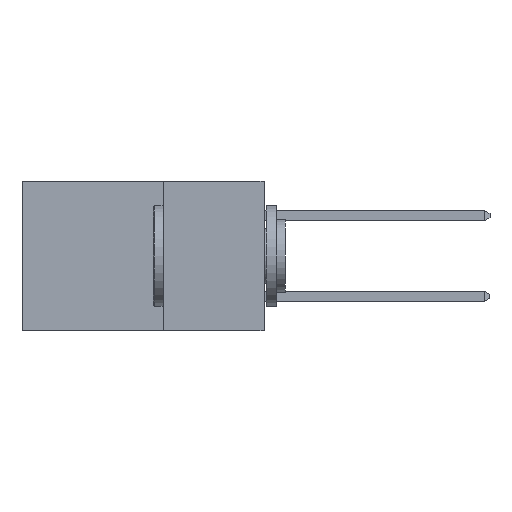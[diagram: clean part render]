
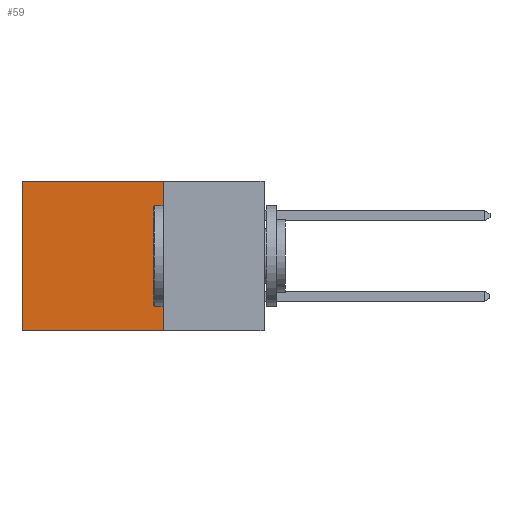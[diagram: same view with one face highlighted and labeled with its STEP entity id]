
A CAD part, left-side view. The second image highlights one B-rep face of the part: STEP entity #59.
In plain terms, the highlighted planar face has unit normal (-1, 0, 0).
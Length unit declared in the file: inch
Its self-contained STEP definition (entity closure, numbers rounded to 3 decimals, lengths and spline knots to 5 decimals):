
#59 = ADVANCED_FACE ( 'NONE', ( #3727 ), #8161, .F. ) ;
#209 = VERTEX_POINT ( 'NONE', #6655 ) ;
#684 = DIRECTION ( 'NONE',  ( 0., 1., 0. ) ) ;
#915 = EDGE_LOOP ( 'NONE', ( #1924, #1939, #1951, #2001 ) ) ;
#956 = VECTOR ( 'NONE', #684, 39.37008 ) ;
#1841 = CARTESIAN_POINT ( 'NONE',  ( 0.298, 0.25, 0. ) ) ;
#1924 = ORIENTED_EDGE ( 'NONE', *, *, #4105, .T. ) ;
#1939 = ORIENTED_EDGE ( 'NONE', *, *, #3051, .F. ) ;
#1951 = ORIENTED_EDGE ( 'NONE', *, *, #7967, .F. ) ;
#2001 = ORIENTED_EDGE ( 'NONE', *, *, #9810, .T. ) ;
#2550 = VECTOR ( 'NONE', #6316, 39.37008 ) ;
#2559 = CARTESIAN_POINT ( 'NONE',  ( 0.298, 0.25, -0.37 ) ) ;
#2726 = VERTEX_POINT ( 'NONE', #8620 ) ;
#3051 = EDGE_CURVE ( 'NONE', #2726, #209, #3172, .T. ) ;
#3147 = LINE ( 'NONE', #5166, #5351 ) ;
#3172 = LINE ( 'NONE', #2559, #956 ) ;
#3714 = AXIS2_PLACEMENT_3D ( 'NONE', #1841, #8182, #6982 ) ;
#3727 = FACE_OUTER_BOUND ( 'NONE', #915, .T. ) ;
#4105 = EDGE_CURVE ( 'NONE', #5704, #209, #6999, .T. ) ;
#4434 = DIRECTION ( 'NONE',  ( 0., 1., 0. ) ) ;
#4798 = LINE ( 'NONE', #9289, #2550 ) ;
#4989 = VECTOR ( 'NONE', #8642, 39.37008 ) ;
#5166 = CARTESIAN_POINT ( 'NONE',  ( 0.298, 0.25, 0. ) ) ;
#5224 = VERTEX_POINT ( 'NONE', #6948 ) ;
#5351 = VECTOR ( 'NONE', #4434, 39.37008 ) ;
#5704 = VERTEX_POINT ( 'NONE', #9781 ) ;
#6316 = DIRECTION ( 'NONE',  ( 0., 0., -1. ) ) ;
#6655 = CARTESIAN_POINT ( 'NONE',  ( 0.298, 0.6, -0.37 ) ) ;
#6948 = CARTESIAN_POINT ( 'NONE',  ( 0.298, 0.25, 0. ) ) ;
#6982 = DIRECTION ( 'NONE',  ( 0., 0., -1. ) ) ;
#6999 = LINE ( 'NONE', #7844, #4989 ) ;
#7844 = CARTESIAN_POINT ( 'NONE',  ( 0.298, 0.6, 0. ) ) ;
#7967 = EDGE_CURVE ( 'NONE', #5224, #2726, #4798, .T. ) ;
#8161 = PLANE ( 'NONE',  #3714 ) ;
#8182 = DIRECTION ( 'NONE',  ( 1., 0., 0. ) ) ;
#8620 = CARTESIAN_POINT ( 'NONE',  ( 0.298, 0.25, -0.37 ) ) ;
#8642 = DIRECTION ( 'NONE',  ( 0., 0., -1. ) ) ;
#9289 = CARTESIAN_POINT ( 'NONE',  ( 0.298, 0.25, 0. ) ) ;
#9781 = CARTESIAN_POINT ( 'NONE',  ( 0.298, 0.6, 0. ) ) ;
#9810 = EDGE_CURVE ( 'NONE', #5224, #5704, #3147, .T. ) ;
